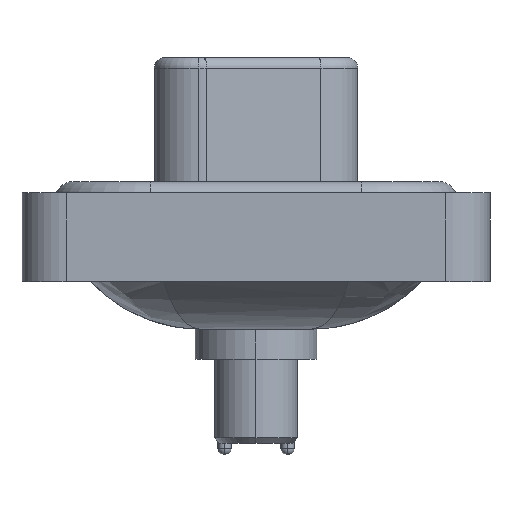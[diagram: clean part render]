
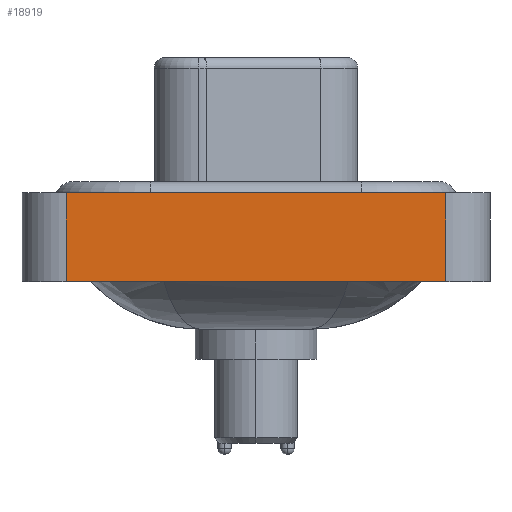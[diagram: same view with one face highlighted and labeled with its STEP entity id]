
A CAD part, left-side view. The second image highlights one B-rep face of the part: STEP entity #18919.
In plain terms, the highlighted planar face has unit normal (-1, 0, 0).
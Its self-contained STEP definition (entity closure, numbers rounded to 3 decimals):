
#156 = VECTOR ( 'NONE', #9344, 1000. ) ;
#548 = ORIENTED_EDGE ( 'NONE', *, *, #15542, .T. ) ;
#643 = CARTESIAN_POINT ( 'NONE',  ( -7.35, -8.55, -3.6 ) ) ;
#1015 = DIRECTION ( 'NONE',  ( -1., 0., 0. ) ) ;
#2608 = CARTESIAN_POINT ( 'NONE',  ( -7.35, 8.55, -3.6 ) ) ;
#3513 = EDGE_CURVE ( 'NONE', #18536, #20235, #15626, .T. ) ;
#4758 = LINE ( 'NONE', #18544, #15365 ) ;
#5279 = CARTESIAN_POINT ( 'NONE',  ( -7.35, 8.55, -3.6 ) ) ;
#5720 = DIRECTION ( 'NONE',  ( 0., -1., 0. ) ) ;
#5880 = CARTESIAN_POINT ( 'NONE',  ( -7.35, -8.55, -3.6 ) ) ;
#6804 = AXIS2_PLACEMENT_3D ( 'NONE', #5880, #1015, #18004 ) ;
#7150 = ORIENTED_EDGE ( 'NONE', *, *, #3513, .F. ) ;
#7608 = LINE ( 'NONE', #643, #20898 ) ;
#8683 = EDGE_CURVE ( 'NONE', #20235, #13779, #4758, .T. ) ;
#9344 = DIRECTION ( 'NONE',  ( 0., 0., 1. ) ) ;
#10072 = LINE ( 'NONE', #16787, #17738 ) ;
#10172 = DIRECTION ( 'NONE',  ( 0., -1., 0. ) ) ;
#10925 = CARTESIAN_POINT ( 'NONE',  ( -7.35, -8.55, -3.6 ) ) ;
#10953 = FACE_OUTER_BOUND ( 'NONE', #17999, .T. ) ;
#11303 = CARTESIAN_POINT ( 'NONE',  ( -7.35, 8.55, 0.4 ) ) ;
#13118 = CARTESIAN_POINT ( 'NONE',  ( -7.35, -8.55, 0.4 ) ) ;
#13693 = VERTEX_POINT ( 'NONE', #10925 ) ;
#13779 = VERTEX_POINT ( 'NONE', #13118 ) ;
#14587 = PLANE ( 'NONE',  #6804 ) ;
#14869 = ORIENTED_EDGE ( 'NONE', *, *, #8683, .F. ) ;
#15365 = VECTOR ( 'NONE', #10172, 1000. ) ;
#15542 = EDGE_CURVE ( 'NONE', #18536, #13693, #7608, .T. ) ;
#15626 = LINE ( 'NONE', #2608, #156 ) ;
#15768 = EDGE_CURVE ( 'NONE', #13693, #13779, #10072, .T. ) ;
#16787 = CARTESIAN_POINT ( 'NONE',  ( -7.35, -8.55, -3.6 ) ) ;
#17738 = VECTOR ( 'NONE', #20323, 1000. ) ;
#17999 = EDGE_LOOP ( 'NONE', ( #20820, #14869, #7150, #548 ) ) ;
#18004 = DIRECTION ( 'NONE',  ( 0., 0., 1. ) ) ;
#18536 = VERTEX_POINT ( 'NONE', #5279 ) ;
#18544 = CARTESIAN_POINT ( 'NONE',  ( -7.35, -8.55, 0.4 ) ) ;
#18919 = ADVANCED_FACE ( 'NONE', ( #10953 ), #14587, .T. ) ;
#20235 = VERTEX_POINT ( 'NONE', #11303 ) ;
#20323 = DIRECTION ( 'NONE',  ( 0., 0., 1. ) ) ;
#20820 = ORIENTED_EDGE ( 'NONE', *, *, #15768, .T. ) ;
#20898 = VECTOR ( 'NONE', #5720, 1000. ) ;
